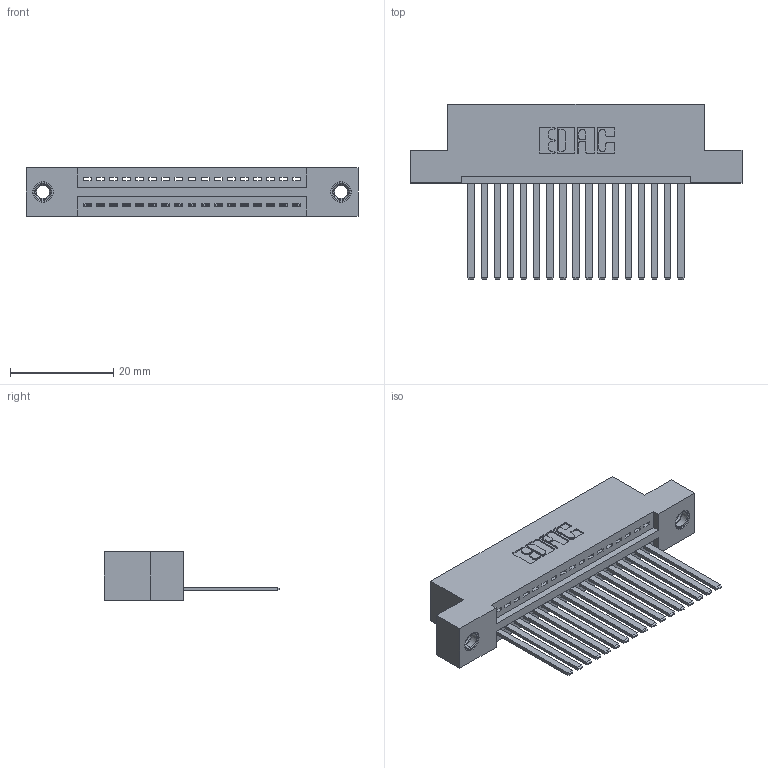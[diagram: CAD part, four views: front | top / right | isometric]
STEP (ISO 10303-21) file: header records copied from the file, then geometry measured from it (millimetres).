
FILE_DESCRIPTION (( 'STEP AP203' ), '1' );
FILE_NAME ('345-017-544-107.STEP', '2019-10-04T16:17:59', ( '' ), ( '' ), 'SwSTEP 2.0', 'SolidWorks 2016', '' );
FILE_SCHEMA (( 'CONFIG_CONTROL_DESIGN' ));
Length unit declared in the file: inch
Products named in the file (4): 345 Part_Flush Mounting Lugs - 0.156 Dia-TI; 345-250-001_345-250-005-103; 345-017-544-107; 345-292-001_345-293-144
Assembly tree (20 placements, depth 2):
  345-017-544-107
    345 Part_Flush Mounting Lugs - 0.156 Dia-TI
    345-292-001_345-293-144  x17
    345-250-001_345-250-005-103  x2
Bounding box: 64.39 x 33.96 x 9.4 mm (x, y, z)
Volume: 6094.3 mm3; surface area: 8382.6 mm2
Topology: 20 solids, 20 shells, 1070 faces, 3163 edges, 2078 vertices
Faces by surface type: plane 724, cylinder 330, cone 12, torus 4
Entity records: 17162 total; most frequent: CARTESIAN_POINT 2954, ORIENTED_EDGE 2898, DIRECTION 2641, EDGE_CURVE 1449, LINE 1233, VECTOR 1233, VERTEX_POINT 960, AXIS2_PLACEMENT_3D 704
